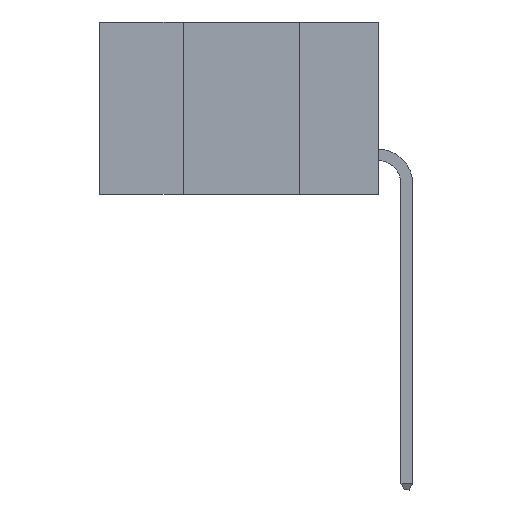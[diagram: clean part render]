
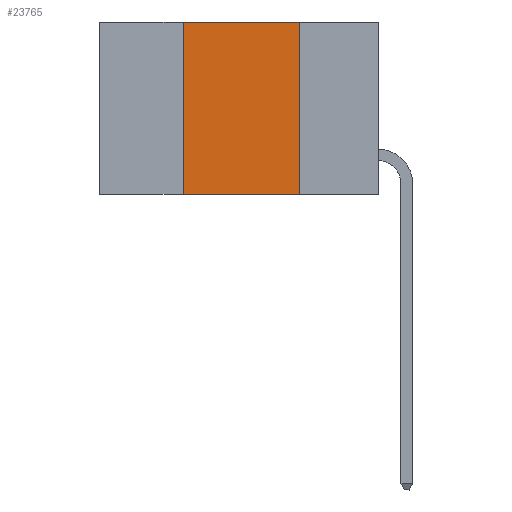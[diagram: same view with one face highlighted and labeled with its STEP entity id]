
A CAD part, left-side view. The second image highlights one B-rep face of the part: STEP entity #23765.
In plain terms, the highlighted planar face has unit normal (-1, 0, 0).
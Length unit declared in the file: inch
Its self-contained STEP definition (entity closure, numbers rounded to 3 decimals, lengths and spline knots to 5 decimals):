
#2504 = VERTEX_POINT ( 'NONE', #26148 ) ;
#3358 = EDGE_CURVE ( 'NONE', #2504, #29167, #16800, .T. ) ;
#4054 = CARTESIAN_POINT ( 'NONE',  ( 0., 0.42, -0.37 ) ) ;
#4587 = DIRECTION ( 'NONE',  ( 1., 0., 0. ) ) ;
#4681 = PLANE ( 'NONE',  #19069 ) ;
#5498 = VERTEX_POINT ( 'NONE', #4054 ) ;
#7137 = CARTESIAN_POINT ( 'NONE',  ( 0., 0.17, 0. ) ) ;
#9404 = LINE ( 'NONE', #7137, #24914 ) ;
#9940 = EDGE_CURVE ( 'NONE', #5498, #2504, #29160, .T. ) ;
#11239 = VERTEX_POINT ( 'NONE', #22299 ) ;
#11286 = LINE ( 'NONE', #26311, #16985 ) ;
#11788 = DIRECTION ( 'NONE',  ( 0., -1., 0. ) ) ;
#12334 = DIRECTION ( 'NONE',  ( 0., 0., -1. ) ) ;
#12453 = ORIENTED_EDGE ( 'NONE', *, *, #25868, .F. ) ;
#12939 = FACE_OUTER_BOUND ( 'NONE', #28412, .T. ) ;
#13330 = ORIENTED_EDGE ( 'NONE', *, *, #9940, .F. ) ;
#13837 = DIRECTION ( 'NONE',  ( 0., 0., 1. ) ) ;
#14732 = CARTESIAN_POINT ( 'NONE',  ( 0., 0.6, 0. ) ) ;
#16786 = DIRECTION ( 'NONE',  ( 0., -1., 0. ) ) ;
#16800 = LINE ( 'NONE', #31298, #23624 ) ;
#16970 = EDGE_CURVE ( 'NONE', #5498, #11239, #11286, .T. ) ;
#16985 = VECTOR ( 'NONE', #11788, 39.37008 ) ;
#18936 = ORIENTED_EDGE ( 'NONE', *, *, #16970, .T. ) ;
#19069 = AXIS2_PLACEMENT_3D ( 'NONE', #14732, #4587, #23975 ) ;
#21427 = CARTESIAN_POINT ( 'NONE',  ( 0., 0.42, 0. ) ) ;
#22299 = CARTESIAN_POINT ( 'NONE',  ( 0., 0.17, -0.37 ) ) ;
#23624 = VECTOR ( 'NONE', #16786, 39.37008 ) ;
#23765 = ADVANCED_FACE ( 'NONE', ( #12939 ), #4681, .F. ) ;
#23975 = DIRECTION ( 'NONE',  ( 0., 0., -1. ) ) ;
#24914 = VECTOR ( 'NONE', #12334, 39.37008 ) ;
#25868 = EDGE_CURVE ( 'NONE', #29167, #11239, #9404, .T. ) ;
#26148 = CARTESIAN_POINT ( 'NONE',  ( 0., 0.42, 0. ) ) ;
#26311 = CARTESIAN_POINT ( 'NONE',  ( 0., 0.6, -0.37 ) ) ;
#28025 = VECTOR ( 'NONE', #13837, 39.37008 ) ;
#28395 = ORIENTED_EDGE ( 'NONE', *, *, #3358, .F. ) ;
#28412 = EDGE_LOOP ( 'NONE', ( #12453, #28395, #13330, #18936 ) ) ;
#29160 = LINE ( 'NONE', #21427, #28025 ) ;
#29167 = VERTEX_POINT ( 'NONE', #30231 ) ;
#30231 = CARTESIAN_POINT ( 'NONE',  ( 0., 0.17, 0. ) ) ;
#31298 = CARTESIAN_POINT ( 'NONE',  ( 0., 0.6, 0. ) ) ;
